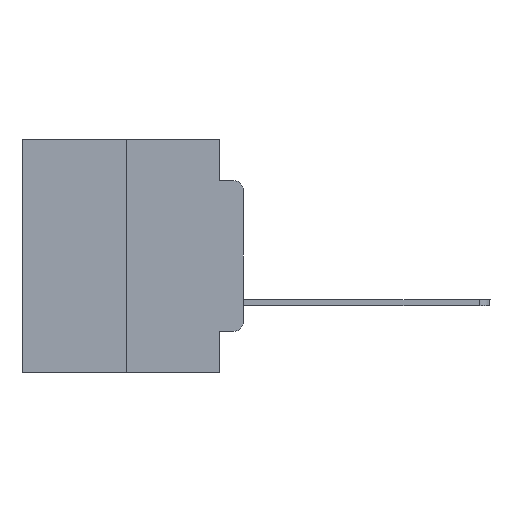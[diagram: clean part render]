
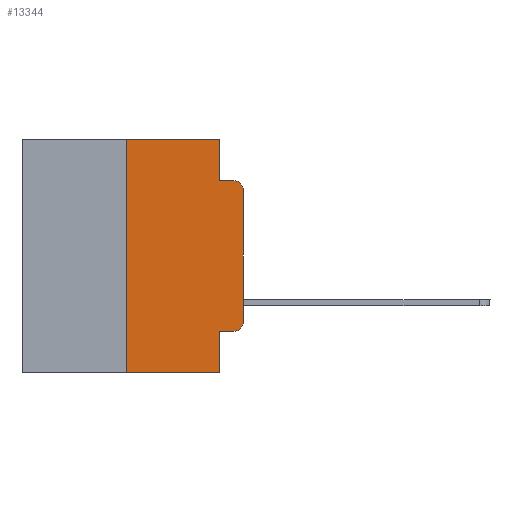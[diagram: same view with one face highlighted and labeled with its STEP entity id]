
A CAD part, left-side view. The second image highlights one B-rep face of the part: STEP entity #13344.
In plain terms, the highlighted planar face has unit normal (-1, 0, 0).
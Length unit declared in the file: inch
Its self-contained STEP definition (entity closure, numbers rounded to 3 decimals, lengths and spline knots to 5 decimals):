
#79 = VERTEX_POINT ( 'NONE', #14047 ) ;
#153 = EDGE_CURVE ( 'NONE', #12957, #25078, #5964, .T. ) ;
#189 = LINE ( 'NONE', #17340, #18203 ) ;
#200 = VERTEX_POINT ( 'NONE', #24470 ) ;
#471 = CARTESIAN_POINT ( 'NONE',  ( 0., 0.25, 0. ) ) ;
#614 = LINE ( 'NONE', #17256, #21113 ) ;
#695 = CARTESIAN_POINT ( 'NONE',  ( 0., 0.02, -0.1085 ) ) ;
#784 = CARTESIAN_POINT ( 'NONE',  ( 0., 0.051, -0.0885 ) ) ;
#1440 = VERTEX_POINT ( 'NONE', #25455 ) ;
#1459 = EDGE_CURVE ( 'NONE', #1440, #21036, #614, .T. ) ;
#1614 = DIRECTION ( 'NONE',  ( 0., 0., -1. ) ) ;
#2126 = CARTESIAN_POINT ( 'NONE',  ( 0., 0.02, -0.4115 ) ) ;
#2222 = AXIS2_PLACEMENT_3D ( 'NONE', #7602, #22062, #1614 ) ;
#2581 = CARTESIAN_POINT ( 'NONE',  ( 0., 0.051, 0. ) ) ;
#2816 = DIRECTION ( 'NONE',  ( 0., -1., 0. ) ) ;
#2931 = EDGE_LOOP ( 'NONE', ( #11295, #16795, #18597, #10899, #18284, #5801, #19644, #4626, #22741, #19397 ) ) ;
#2954 = LINE ( 'NONE', #471, #18447 ) ;
#3003 = AXIS2_PLACEMENT_3D ( 'NONE', #695, #6687, #19032 ) ;
#3111 = PLANE ( 'NONE',  #18483 ) ;
#3920 = VERTEX_POINT ( 'NONE', #2126 ) ;
#3999 = EDGE_CURVE ( 'NONE', #200, #3920, #21566, .T. ) ;
#4626 = ORIENTED_EDGE ( 'NONE', *, *, #15524, .F. ) ;
#5031 = VECTOR ( 'NONE', #20691, 39.37008 ) ;
#5188 = FACE_OUTER_BOUND ( 'NONE', #2931, .T. ) ;
#5459 = VERTEX_POINT ( 'NONE', #14000 ) ;
#5735 = VECTOR ( 'NONE', #21945, 39.37008 ) ;
#5801 = ORIENTED_EDGE ( 'NONE', *, *, #17074, .F. ) ;
#5964 = LINE ( 'NONE', #12727, #5031 ) ;
#6687 = DIRECTION ( 'NONE',  ( -1., 0., 0. ) ) ;
#6913 = VERTEX_POINT ( 'NONE', #24277 ) ;
#7062 = CIRCLE ( 'NONE', #2222, 0.02 ) ;
#7602 = CARTESIAN_POINT ( 'NONE',  ( 0., 0.02, -0.3915 ) ) ;
#8179 = CARTESIAN_POINT ( 'NONE',  ( 0., 0.051, -0.4115 ) ) ;
#9093 = DIRECTION ( 'NONE',  ( 1., 0., 0. ) ) ;
#10473 = DIRECTION ( 'NONE',  ( 0., 0., 1. ) ) ;
#10899 = ORIENTED_EDGE ( 'NONE', *, *, #16041, .F. ) ;
#11067 = EDGE_CURVE ( 'NONE', #21036, #6913, #13679, .T. ) ;
#11295 = ORIENTED_EDGE ( 'NONE', *, *, #1459, .T. ) ;
#12727 = CARTESIAN_POINT ( 'NONE',  ( 0., 0.473, 0. ) ) ;
#12957 = VERTEX_POINT ( 'NONE', #15355 ) ;
#13344 = ADVANCED_FACE ( 'NONE', ( #5188 ), #3111, .F. ) ;
#13410 = LINE ( 'NONE', #23863, #14634 ) ;
#13452 = CARTESIAN_POINT ( 'NONE',  ( 0., 0.051, -0.0885 ) ) ;
#13679 = CIRCLE ( 'NONE', #3003, 0.02 ) ;
#14000 = CARTESIAN_POINT ( 'NONE',  ( 0., 0.051, -0.5 ) ) ;
#14047 = CARTESIAN_POINT ( 'NONE',  ( 0., 0.25, -0.5 ) ) ;
#14634 = VECTOR ( 'NONE', #23778, 39.37008 ) ;
#15355 = CARTESIAN_POINT ( 'NONE',  ( 0., 0.25, 0. ) ) ;
#15524 = EDGE_CURVE ( 'NONE', #200, #5459, #25014, .T. ) ;
#16041 = EDGE_CURVE ( 'NONE', #25078, #19873, #189, .T. ) ;
#16614 = CARTESIAN_POINT ( 'NONE',  ( 0., 0.051, 0. ) ) ;
#16795 = ORIENTED_EDGE ( 'NONE', *, *, #11067, .T. ) ;
#17074 = EDGE_CURVE ( 'NONE', #79, #12957, #2954, .T. ) ;
#17256 = CARTESIAN_POINT ( 'NONE',  ( 0., 0., 0. ) ) ;
#17340 = CARTESIAN_POINT ( 'NONE',  ( 0., 0.051, 0. ) ) ;
#18203 = VECTOR ( 'NONE', #23462, 39.37008 ) ;
#18284 = ORIENTED_EDGE ( 'NONE', *, *, #153, .F. ) ;
#18288 = DIRECTION ( 'NONE',  ( 0., 0., -1. ) ) ;
#18447 = VECTOR ( 'NONE', #10473, 39.37008 ) ;
#18483 = AXIS2_PLACEMENT_3D ( 'NONE', #20945, #9093, #24920 ) ;
#18553 = EDGE_CURVE ( 'NONE', #79, #5459, #13410, .T. ) ;
#18597 = ORIENTED_EDGE ( 'NONE', *, *, #24871, .F. ) ;
#19032 = DIRECTION ( 'NONE',  ( 0., 0., -1. ) ) ;
#19397 = ORIENTED_EDGE ( 'NONE', *, *, #25456, .T. ) ;
#19644 = ORIENTED_EDGE ( 'NONE', *, *, #18553, .T. ) ;
#19873 = VERTEX_POINT ( 'NONE', #13452 ) ;
#20691 = DIRECTION ( 'NONE',  ( 0., -1., 0. ) ) ;
#20703 = LINE ( 'NONE', #784, #25672 ) ;
#20945 = CARTESIAN_POINT ( 'NONE',  ( 0., 0.473, 0. ) ) ;
#21036 = VERTEX_POINT ( 'NONE', #22960 ) ;
#21113 = VECTOR ( 'NONE', #21315, 39.37008 ) ;
#21315 = DIRECTION ( 'NONE',  ( 0., 0., 1. ) ) ;
#21566 = LINE ( 'NONE', #8179, #5735 ) ;
#21945 = DIRECTION ( 'NONE',  ( 0., -1., 0. ) ) ;
#22062 = DIRECTION ( 'NONE',  ( -1., 0., 0. ) ) ;
#22241 = VECTOR ( 'NONE', #18288, 39.37008 ) ;
#22741 = ORIENTED_EDGE ( 'NONE', *, *, #3999, .T. ) ;
#22960 = CARTESIAN_POINT ( 'NONE',  ( 0., 0., -0.1085 ) ) ;
#23462 = DIRECTION ( 'NONE',  ( 0., 0., -1. ) ) ;
#23778 = DIRECTION ( 'NONE',  ( 0., -1., 0. ) ) ;
#23863 = CARTESIAN_POINT ( 'NONE',  ( 0., 0.473, -0.5 ) ) ;
#24277 = CARTESIAN_POINT ( 'NONE',  ( 0., 0.02, -0.0885 ) ) ;
#24470 = CARTESIAN_POINT ( 'NONE',  ( 0., 0.051, -0.4115 ) ) ;
#24871 = EDGE_CURVE ( 'NONE', #19873, #6913, #20703, .T. ) ;
#24920 = DIRECTION ( 'NONE',  ( 0., 0., -1. ) ) ;
#25014 = LINE ( 'NONE', #16614, #22241 ) ;
#25078 = VERTEX_POINT ( 'NONE', #2581 ) ;
#25455 = CARTESIAN_POINT ( 'NONE',  ( 0., 0., -0.3915 ) ) ;
#25456 = EDGE_CURVE ( 'NONE', #3920, #1440, #7062, .T. ) ;
#25672 = VECTOR ( 'NONE', #2816, 39.37008 ) ;
